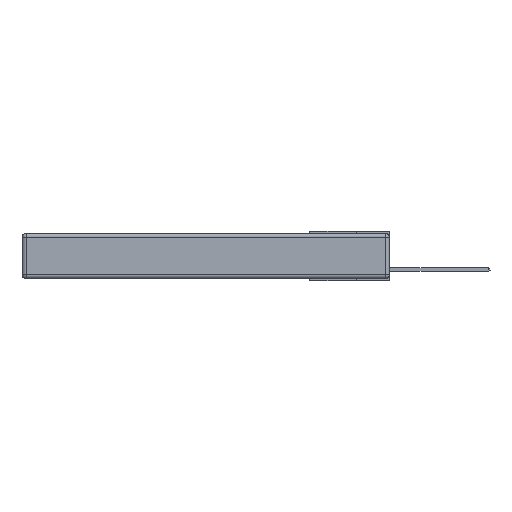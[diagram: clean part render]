
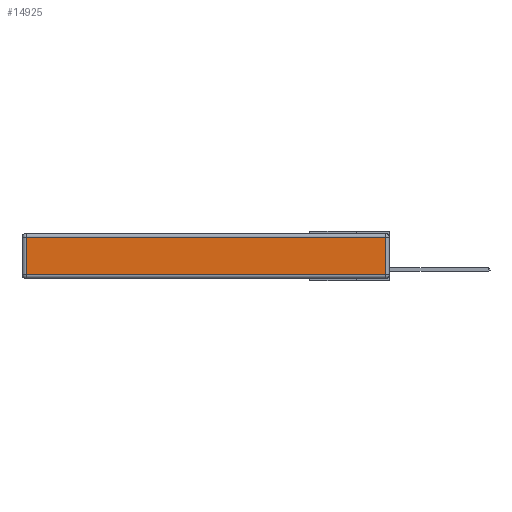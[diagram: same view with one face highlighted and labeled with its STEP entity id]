
A CAD part, left-side view. The second image highlights one B-rep face of the part: STEP entity #14925.
In plain terms, the highlighted planar face has unit normal (-1, 0, 0).
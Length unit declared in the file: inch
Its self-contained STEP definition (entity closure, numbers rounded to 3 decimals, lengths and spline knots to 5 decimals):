
#408 = VECTOR ( 'NONE', #10670, 39.37008 ) ;
#680 = DIRECTION ( 'NONE',  ( -1., 0., 0. ) ) ;
#841 = CARTESIAN_POINT ( 'NONE',  ( 0., 0., -0.343 ) ) ;
#1485 = LINE ( 'NONE', #23590, #23888 ) ;
#2078 = ORIENTED_EDGE ( 'NONE', *, *, #6276, .T. ) ;
#2699 = LINE ( 'NONE', #10301, #9111 ) ;
#6137 = CARTESIAN_POINT ( 'NONE',  ( 0., 2.72, -0.313 ) ) ;
#6276 = EDGE_CURVE ( 'NONE', #18007, #11193, #19042, .T. ) ;
#6493 = AXIS2_PLACEMENT_3D ( 'NONE', #841, #680, #12521 ) ;
#7630 = FACE_OUTER_BOUND ( 'NONE', #15819, .T. ) ;
#8804 = CARTESIAN_POINT ( 'NONE',  ( 0., 2.72, -0.03 ) ) ;
#9111 = VECTOR ( 'NONE', #19990, 39.37008 ) ;
#9885 = EDGE_CURVE ( 'NONE', #11193, #20457, #2699, .T. ) ;
#9942 = DIRECTION ( 'NONE',  ( 0., 0., 1. ) ) ;
#10126 = VECTOR ( 'NONE', #16684, 39.37008 ) ;
#10301 = CARTESIAN_POINT ( 'NONE',  ( 0., 2.72, -0.343 ) ) ;
#10670 = DIRECTION ( 'NONE',  ( 0., -1., 0. ) ) ;
#11161 = ORIENTED_EDGE ( 'NONE', *, *, #19488, .T. ) ;
#11193 = VERTEX_POINT ( 'NONE', #8804 ) ;
#11227 = CARTESIAN_POINT ( 'NONE',  ( 0., 0.03, -0.03 ) ) ;
#12119 = EDGE_CURVE ( 'NONE', #20457, #16336, #20339, .T. ) ;
#12521 = DIRECTION ( 'NONE',  ( 0., 0., 1. ) ) ;
#12602 = PLANE ( 'NONE',  #6493 ) ;
#14925 = ADVANCED_FACE ( 'NONE', ( #7630 ), #12602, .T. ) ;
#15819 = EDGE_LOOP ( 'NONE', ( #19169, #11161, #2078, #21201 ) ) ;
#16336 = VERTEX_POINT ( 'NONE', #17212 ) ;
#16684 = DIRECTION ( 'NONE',  ( 0., 1., 0. ) ) ;
#17212 = CARTESIAN_POINT ( 'NONE',  ( 0., 0.03, -0.313 ) ) ;
#18007 = VERTEX_POINT ( 'NONE', #11227 ) ;
#19042 = LINE ( 'NONE', #20530, #10126 ) ;
#19169 = ORIENTED_EDGE ( 'NONE', *, *, #12119, .T. ) ;
#19488 = EDGE_CURVE ( 'NONE', #16336, #18007, #1485, .T. ) ;
#19990 = DIRECTION ( 'NONE',  ( 0., 0., -1. ) ) ;
#20339 = LINE ( 'NONE', #24141, #408 ) ;
#20457 = VERTEX_POINT ( 'NONE', #6137 ) ;
#20530 = CARTESIAN_POINT ( 'NONE',  ( 0., 2.75, -0.03 ) ) ;
#21201 = ORIENTED_EDGE ( 'NONE', *, *, #9885, .T. ) ;
#23590 = CARTESIAN_POINT ( 'NONE',  ( 0., 0.03, -0.343 ) ) ;
#23888 = VECTOR ( 'NONE', #9942, 39.37008 ) ;
#24141 = CARTESIAN_POINT ( 'NONE',  ( 0., 0., -0.313 ) ) ;
